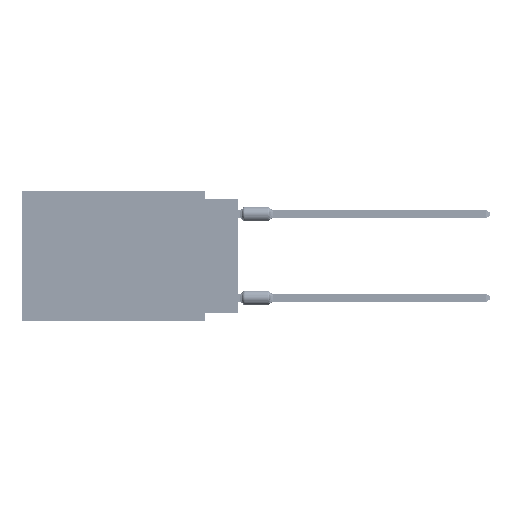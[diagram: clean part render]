
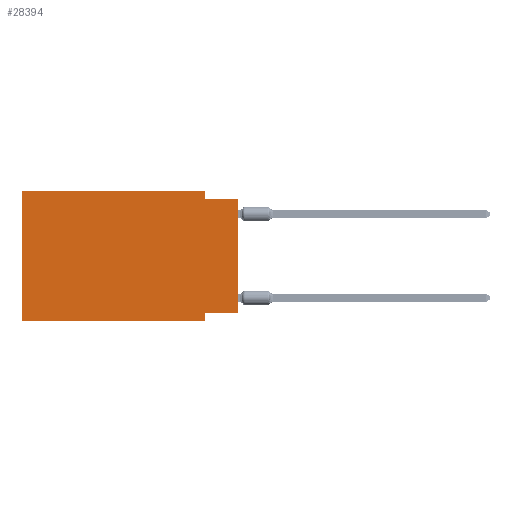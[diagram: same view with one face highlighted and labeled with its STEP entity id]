
A CAD part, left-side view. The second image highlights one B-rep face of the part: STEP entity #28394.
In plain terms, the highlighted planar face has unit normal (-1, 0, 0).
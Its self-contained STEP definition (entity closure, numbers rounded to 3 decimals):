
#21 = CARTESIAN_POINT ( 'NONE',  ( 0., 16.383, -9.906 ) ) ;
#1758 = EDGE_CURVE ( 'NONE', #8568, #40272, #15084, .T. ) ;
#2081 = CARTESIAN_POINT ( 'NONE',  ( 0., 16.383, 0. ) ) ;
#3411 = LINE ( 'NONE', #77198, #54996 ) ;
#3996 = VECTOR ( 'NONE', #38561, 1000. ) ;
#6641 = CARTESIAN_POINT ( 'NONE',  ( 0., 0., -0.635 ) ) ;
#7639 = VECTOR ( 'NONE', #68429, 1000. ) ;
#8568 = VERTEX_POINT ( 'NONE', #11518 ) ;
#9566 = ORIENTED_EDGE ( 'NONE', *, *, #72336, .F. ) ;
#9877 = EDGE_CURVE ( 'NONE', #8568, #11815, #42369, .T. ) ;
#11518 = CARTESIAN_POINT ( 'NONE',  ( 0., 16.383, -9.906 ) ) ;
#11815 = VERTEX_POINT ( 'NONE', #24852 ) ;
#14211 = CARTESIAN_POINT ( 'NONE',  ( 0., 2.54, 0. ) ) ;
#14820 = EDGE_CURVE ( 'NONE', #40272, #39994, #31083, .T. ) ;
#15084 = LINE ( 'NONE', #76056, #73266 ) ;
#15487 = VECTOR ( 'NONE', #72224, 1000. ) ;
#17485 = DIRECTION ( 'NONE',  ( 0., -1., 0. ) ) ;
#17888 = CARTESIAN_POINT ( 'NONE',  ( 0., 16.383, 0. ) ) ;
#20047 = VERTEX_POINT ( 'NONE', #37516 ) ;
#22069 = AXIS2_PLACEMENT_3D ( 'NONE', #24161, #66812, #72770 ) ;
#23811 = ORIENTED_EDGE ( 'NONE', *, *, #1758, .F. ) ;
#24161 = CARTESIAN_POINT ( 'NONE',  ( 0., 16.383, 0. ) ) ;
#24852 = CARTESIAN_POINT ( 'NONE',  ( 0., 2.54, -9.906 ) ) ;
#24885 = VERTEX_POINT ( 'NONE', #35933 ) ;
#25483 = ORIENTED_EDGE ( 'NONE', *, *, #61833, .F. ) ;
#25656 = CARTESIAN_POINT ( 'NONE',  ( 0., 2.54, -9.271 ) ) ;
#26173 = LINE ( 'NONE', #6641, #7639 ) ;
#28394 = ADVANCED_FACE ( 'NONE', ( #78737 ), #41343, .F. ) ;
#31083 = LINE ( 'NONE', #17888, #39587 ) ;
#34292 = CARTESIAN_POINT ( 'NONE',  ( 0., 0., -9.271 ) ) ;
#34585 = DIRECTION ( 'NONE',  ( 0., 0., -1. ) ) ;
#34979 = CARTESIAN_POINT ( 'NONE',  ( 0., 2.54, -0.635 ) ) ;
#35083 = LINE ( 'NONE', #34292, #53781 ) ;
#35933 = CARTESIAN_POINT ( 'NONE',  ( 0., 0., -9.271 ) ) ;
#37516 = CARTESIAN_POINT ( 'NONE',  ( 0., 0., -0.635 ) ) ;
#38561 = DIRECTION ( 'NONE',  ( 0., 0., -1. ) ) ;
#39470 = ORIENTED_EDGE ( 'NONE', *, *, #41486, .F. ) ;
#39587 = VECTOR ( 'NONE', #17485, 1000. ) ;
#39994 = VERTEX_POINT ( 'NONE', #48045 ) ;
#40272 = VERTEX_POINT ( 'NONE', #2081 ) ;
#41343 = PLANE ( 'NONE',  #22069 ) ;
#41486 = EDGE_CURVE ( 'NONE', #39994, #52135, #69239, .T. ) ;
#42369 = LINE ( 'NONE', #21, #15487 ) ;
#44112 = LINE ( 'NONE', #61659, #64641 ) ;
#46198 = DIRECTION ( 'NONE',  ( 0., 0., 1. ) ) ;
#48045 = CARTESIAN_POINT ( 'NONE',  ( 0., 2.54, 0. ) ) ;
#48784 = ORIENTED_EDGE ( 'NONE', *, *, #50056, .T. ) ;
#48818 = EDGE_LOOP ( 'NONE', ( #48784, #9566, #39470, #55083, #23811, #70945, #68604, #25483 ) ) ;
#50056 = EDGE_CURVE ( 'NONE', #24885, #20047, #44112, .T. ) ;
#52135 = VERTEX_POINT ( 'NONE', #34979 ) ;
#53781 = VECTOR ( 'NONE', #65756, 1000. ) ;
#54996 = VECTOR ( 'NONE', #34585, 1000. ) ;
#55083 = ORIENTED_EDGE ( 'NONE', *, *, #14820, .F. ) ;
#61659 = CARTESIAN_POINT ( 'NONE',  ( 0., 0., 0. ) ) ;
#61833 = EDGE_CURVE ( 'NONE', #24885, #74191, #35083, .T. ) ;
#64641 = VECTOR ( 'NONE', #73182, 1000. ) ;
#65756 = DIRECTION ( 'NONE',  ( 0., 1., 0. ) ) ;
#66812 = DIRECTION ( 'NONE',  ( 1., 0., 0. ) ) ;
#68429 = DIRECTION ( 'NONE',  ( 0., -1., 0. ) ) ;
#68604 = ORIENTED_EDGE ( 'NONE', *, *, #74693, .F. ) ;
#69239 = LINE ( 'NONE', #14211, #3996 ) ;
#70945 = ORIENTED_EDGE ( 'NONE', *, *, #9877, .T. ) ;
#72224 = DIRECTION ( 'NONE',  ( 0., -1., 0. ) ) ;
#72336 = EDGE_CURVE ( 'NONE', #52135, #20047, #26173, .T. ) ;
#72770 = DIRECTION ( 'NONE',  ( 0., 0., -1. ) ) ;
#73182 = DIRECTION ( 'NONE',  ( 0., 0., 1. ) ) ;
#73266 = VECTOR ( 'NONE', #46198, 1000. ) ;
#74191 = VERTEX_POINT ( 'NONE', #25656 ) ;
#74693 = EDGE_CURVE ( 'NONE', #74191, #11815, #3411, .T. ) ;
#76056 = CARTESIAN_POINT ( 'NONE',  ( 0., 16.383, 0. ) ) ;
#77198 = CARTESIAN_POINT ( 'NONE',  ( 0., 2.54, -9.906 ) ) ;
#78737 = FACE_OUTER_BOUND ( 'NONE', #48818, .T. ) ;
